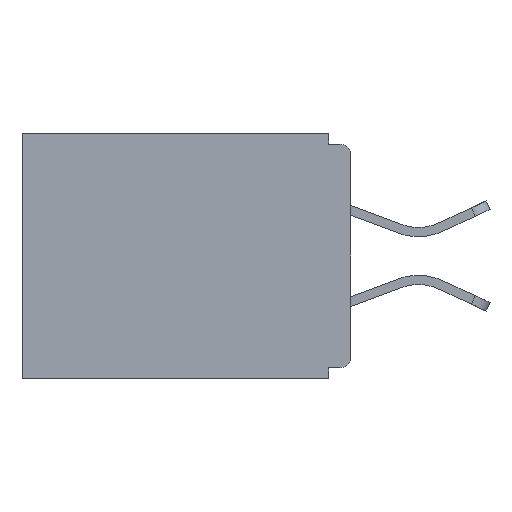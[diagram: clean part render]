
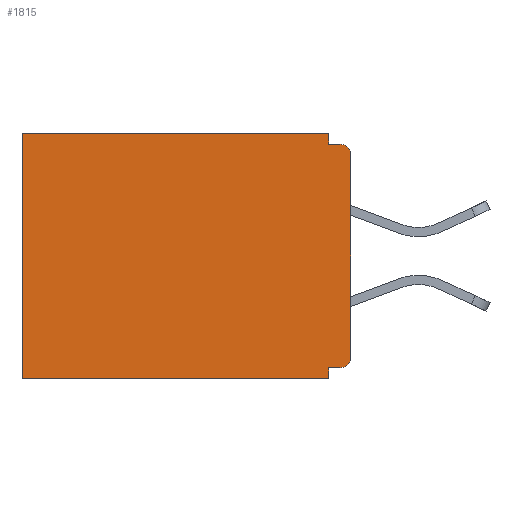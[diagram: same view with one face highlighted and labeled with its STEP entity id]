
A CAD part, left-side view. The second image highlights one B-rep face of the part: STEP entity #1815.
In plain terms, the highlighted planar face has unit normal (-1, 0, 0).
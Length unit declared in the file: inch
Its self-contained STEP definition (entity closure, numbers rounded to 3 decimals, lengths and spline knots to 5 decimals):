
#62 = ORIENTED_EDGE ( 'NONE', *, *, #7968, .F. ) ;
#116 = CARTESIAN_POINT ( 'NONE',  ( 0.298, 0.015, -0.015 ) ) ;
#263 = ORIENTED_EDGE ( 'NONE', *, *, #4718, .T. ) ;
#286 = ORIENTED_EDGE ( 'NONE', *, *, #4194, .F. ) ;
#364 = CARTESIAN_POINT ( 'NONE',  ( 0.298, 0.031, -0.343 ) ) ;
#481 = LINE ( 'NONE', #4670, #10687 ) ;
#561 = AXIS2_PLACEMENT_3D ( 'NONE', #1276, #1164, #5482 ) ;
#695 = CARTESIAN_POINT ( 'NONE',  ( 0.298, 0., 0. ) ) ;
#732 = DIRECTION ( 'NONE',  ( 0., 1., 0. ) ) ;
#838 = CARTESIAN_POINT ( 'NONE',  ( 0.298, 0.46, 0. ) ) ;
#940 = CARTESIAN_POINT ( 'NONE',  ( 0.298, 0., -0.313 ) ) ;
#1028 = CARTESIAN_POINT ( 'NONE',  ( 0.298, 0.031, -0.343 ) ) ;
#1110 = VERTEX_POINT ( 'NONE', #2127 ) ;
#1164 = DIRECTION ( 'NONE',  ( -1., 0., 0. ) ) ;
#1276 = CARTESIAN_POINT ( 'NONE',  ( 0.298, 0.015, -0.313 ) ) ;
#1375 = VECTOR ( 'NONE', #7909, 39.37008 ) ;
#1695 = VECTOR ( 'NONE', #9146, 39.37008 ) ;
#1769 = LINE ( 'NONE', #2515, #8842 ) ;
#1806 = DIRECTION ( 'NONE',  ( 0., -1., 0. ) ) ;
#1815 = ADVANCED_FACE ( 'NONE', ( #6643 ), #9440, .F. ) ;
#1922 = AXIS2_PLACEMENT_3D ( 'NONE', #10271, #5280, #6121 ) ;
#1959 = VERTEX_POINT ( 'NONE', #10301 ) ;
#2127 = CARTESIAN_POINT ( 'NONE',  ( 0.298, 0.031, -0.015 ) ) ;
#2140 = VERTEX_POINT ( 'NONE', #8001 ) ;
#2177 = EDGE_CURVE ( 'NONE', #3060, #4436, #481, .T. ) ;
#2335 = VERTEX_POINT ( 'NONE', #4964 ) ;
#2515 = CARTESIAN_POINT ( 'NONE',  ( 0.298, 0., -0.015 ) ) ;
#2612 = CIRCLE ( 'NONE', #5515, 0.015 ) ;
#2619 = LINE ( 'NONE', #695, #1695 ) ;
#2904 = EDGE_CURVE ( 'NONE', #1110, #4109, #1769, .T. ) ;
#2954 = LINE ( 'NONE', #838, #4915 ) ;
#3060 = VERTEX_POINT ( 'NONE', #9397 ) ;
#3616 = DIRECTION ( 'NONE',  ( 0., 0., -1. ) ) ;
#3943 = ORIENTED_EDGE ( 'NONE', *, *, #8486, .T. ) ;
#4109 = VERTEX_POINT ( 'NONE', #116 ) ;
#4194 = EDGE_CURVE ( 'NONE', #2140, #1110, #8428, .T. ) ;
#4436 = VERTEX_POINT ( 'NONE', #8253 ) ;
#4670 = CARTESIAN_POINT ( 'NONE',  ( 0.298, 0., -0.328 ) ) ;
#4713 = CARTESIAN_POINT ( 'NONE',  ( 0.298, 0., 0. ) ) ;
#4718 = EDGE_CURVE ( 'NONE', #3060, #10534, #10107, .T. ) ;
#4915 = VECTOR ( 'NONE', #9906, 39.37008 ) ;
#4964 = CARTESIAN_POINT ( 'NONE',  ( 0.298, 0., -0.03 ) ) ;
#5189 = DIRECTION ( 'NONE',  ( -1., 0., 0. ) ) ;
#5280 = DIRECTION ( 'NONE',  ( 1., 0., 0. ) ) ;
#5482 = DIRECTION ( 'NONE',  ( 0., 0., -1. ) ) ;
#5515 = AXIS2_PLACEMENT_3D ( 'NONE', #8506, #5189, #6962 ) ;
#5769 = DIRECTION ( 'NONE',  ( 0., 0., -1. ) ) ;
#6121 = DIRECTION ( 'NONE',  ( 0., 0., -1. ) ) ;
#6163 = LINE ( 'NONE', #9837, #8501 ) ;
#6337 = EDGE_CURVE ( 'NONE', #1959, #7034, #6163, .T. ) ;
#6353 = EDGE_CURVE ( 'NONE', #2140, #8317, #2619, .T. ) ;
#6643 = FACE_OUTER_BOUND ( 'NONE', #9947, .T. ) ;
#6694 = ORIENTED_EDGE ( 'NONE', *, *, #2177, .F. ) ;
#6818 = ORIENTED_EDGE ( 'NONE', *, *, #6337, .F. ) ;
#6962 = DIRECTION ( 'NONE',  ( 0., 0., -1. ) ) ;
#7034 = VERTEX_POINT ( 'NONE', #7127 ) ;
#7127 = CARTESIAN_POINT ( 'NONE',  ( 0.298, 0.46, -0.343 ) ) ;
#7174 = ORIENTED_EDGE ( 'NONE', *, *, #7849, .F. ) ;
#7415 = LINE ( 'NONE', #4713, #9770 ) ;
#7465 = ORIENTED_EDGE ( 'NONE', *, *, #10201, .T. ) ;
#7550 = LINE ( 'NONE', #1028, #9897 ) ;
#7849 = EDGE_CURVE ( 'NONE', #4436, #1959, #7550, .T. ) ;
#7909 = DIRECTION ( 'NONE',  ( 0., 0., -1. ) ) ;
#7968 = EDGE_CURVE ( 'NONE', #2335, #10534, #7415, .T. ) ;
#8001 = CARTESIAN_POINT ( 'NONE',  ( 0.298, 0.031, 0. ) ) ;
#8007 = CARTESIAN_POINT ( 'NONE',  ( 0.298, 0.46, 0. ) ) ;
#8253 = CARTESIAN_POINT ( 'NONE',  ( 0.298, 0.031, -0.328 ) ) ;
#8317 = VERTEX_POINT ( 'NONE', #8007 ) ;
#8428 = LINE ( 'NONE', #364, #1375 ) ;
#8486 = EDGE_CURVE ( 'NONE', #8317, #7034, #2954, .T. ) ;
#8501 = VECTOR ( 'NONE', #732, 39.37008 ) ;
#8506 = CARTESIAN_POINT ( 'NONE',  ( 0.298, 0.015, -0.03 ) ) ;
#8690 = ORIENTED_EDGE ( 'NONE', *, *, #6353, .T. ) ;
#8842 = VECTOR ( 'NONE', #1806, 39.37008 ) ;
#8871 = DIRECTION ( 'NONE',  ( 0., 1., 0. ) ) ;
#9146 = DIRECTION ( 'NONE',  ( 0., 1., 0. ) ) ;
#9357 = ORIENTED_EDGE ( 'NONE', *, *, #2904, .F. ) ;
#9397 = CARTESIAN_POINT ( 'NONE',  ( 0.298, 0.015, -0.328 ) ) ;
#9440 = PLANE ( 'NONE',  #1922 ) ;
#9770 = VECTOR ( 'NONE', #5769, 39.37008 ) ;
#9837 = CARTESIAN_POINT ( 'NONE',  ( 0.298, 0., -0.343 ) ) ;
#9897 = VECTOR ( 'NONE', #3616, 39.37008 ) ;
#9906 = DIRECTION ( 'NONE',  ( 0., 0., -1. ) ) ;
#9947 = EDGE_LOOP ( 'NONE', ( #7465, #9357, #286, #8690, #3943, #6818, #7174, #6694, #263, #62 ) ) ;
#10107 = CIRCLE ( 'NONE', #561, 0.015 ) ;
#10201 = EDGE_CURVE ( 'NONE', #2335, #4109, #2612, .T. ) ;
#10271 = CARTESIAN_POINT ( 'NONE',  ( 0.298, 0., 0. ) ) ;
#10301 = CARTESIAN_POINT ( 'NONE',  ( 0.298, 0.031, -0.343 ) ) ;
#10534 = VERTEX_POINT ( 'NONE', #940 ) ;
#10687 = VECTOR ( 'NONE', #8871, 39.37008 ) ;
